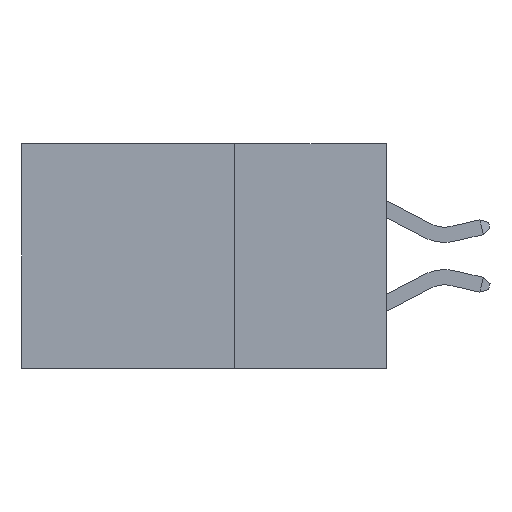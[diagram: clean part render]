
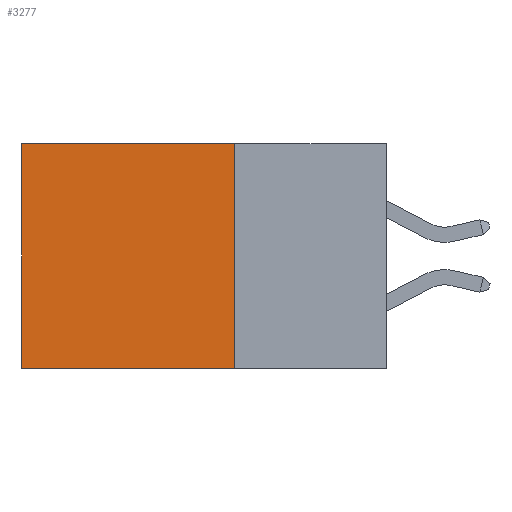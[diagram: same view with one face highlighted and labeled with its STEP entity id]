
A CAD part, left-side view. The second image highlights one B-rep face of the part: STEP entity #3277.
In plain terms, the highlighted planar face has unit normal (-1, 0, 0).
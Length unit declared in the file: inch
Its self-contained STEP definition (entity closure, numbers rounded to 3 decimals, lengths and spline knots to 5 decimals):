
#2470 = ORIENTED_EDGE ( 'NONE', *, *, #12406, .T. ) ;
#3062 = LINE ( 'NONE', #16408, #14953 ) ;
#3147 = EDGE_LOOP ( 'NONE', ( #2470, #16339, #15333, #8683 ) ) ;
#3277 = ADVANCED_FACE ( 'NONE', ( #4657 ), #14425, .F. ) ;
#3490 = CARTESIAN_POINT ( 'NONE',  ( 0.298, 0.6, 0. ) ) ;
#4657 = FACE_OUTER_BOUND ( 'NONE', #3147, .T. ) ;
#4663 = AXIS2_PLACEMENT_3D ( 'NONE', #15683, #17262, #10315 ) ;
#6171 = DIRECTION ( 'NONE',  ( 0., 1., 0. ) ) ;
#6346 = EDGE_CURVE ( 'NONE', #10489, #9769, #13392, .T. ) ;
#6501 = VERTEX_POINT ( 'NONE', #8355 ) ;
#6892 = VECTOR ( 'NONE', #13406, 39.37008 ) ;
#8355 = CARTESIAN_POINT ( 'NONE',  ( 0.298, 0.25, -0.37 ) ) ;
#8665 = LINE ( 'NONE', #16120, #6892 ) ;
#8683 = ORIENTED_EDGE ( 'NONE', *, *, #6346, .T. ) ;
#9316 = CARTESIAN_POINT ( 'NONE',  ( 0.298, 0.25, -0.37 ) ) ;
#9769 = VERTEX_POINT ( 'NONE', #3490 ) ;
#10315 = DIRECTION ( 'NONE',  ( 0., 0., -1. ) ) ;
#10489 = VERTEX_POINT ( 'NONE', #15574 ) ;
#10535 = EDGE_CURVE ( 'NONE', #10489, #6501, #3062, .T. ) ;
#12244 = DIRECTION ( 'NONE',  ( 0., 0., -1. ) ) ;
#12406 = EDGE_CURVE ( 'NONE', #9769, #15964, #8665, .T. ) ;
#13000 = CARTESIAN_POINT ( 'NONE',  ( 0.298, 0.25, 0. ) ) ;
#13106 = LINE ( 'NONE', #9316, #14837 ) ;
#13392 = LINE ( 'NONE', #13000, #15328 ) ;
#13406 = DIRECTION ( 'NONE',  ( 0., 0., -1. ) ) ;
#13497 = DIRECTION ( 'NONE',  ( 0., 1., 0. ) ) ;
#14412 = EDGE_CURVE ( 'NONE', #6501, #15964, #13106, .T. ) ;
#14425 = PLANE ( 'NONE',  #4663 ) ;
#14571 = CARTESIAN_POINT ( 'NONE',  ( 0.298, 0.6, -0.37 ) ) ;
#14837 = VECTOR ( 'NONE', #13497, 39.37008 ) ;
#14953 = VECTOR ( 'NONE', #12244, 39.37008 ) ;
#15328 = VECTOR ( 'NONE', #6171, 39.37008 ) ;
#15333 = ORIENTED_EDGE ( 'NONE', *, *, #10535, .F. ) ;
#15574 = CARTESIAN_POINT ( 'NONE',  ( 0.298, 0.25, 0. ) ) ;
#15683 = CARTESIAN_POINT ( 'NONE',  ( 0.298, 0.25, 0. ) ) ;
#15964 = VERTEX_POINT ( 'NONE', #14571 ) ;
#16120 = CARTESIAN_POINT ( 'NONE',  ( 0.298, 0.6, 0. ) ) ;
#16339 = ORIENTED_EDGE ( 'NONE', *, *, #14412, .F. ) ;
#16408 = CARTESIAN_POINT ( 'NONE',  ( 0.298, 0.25, 0. ) ) ;
#17262 = DIRECTION ( 'NONE',  ( 1., 0., 0. ) ) ;
